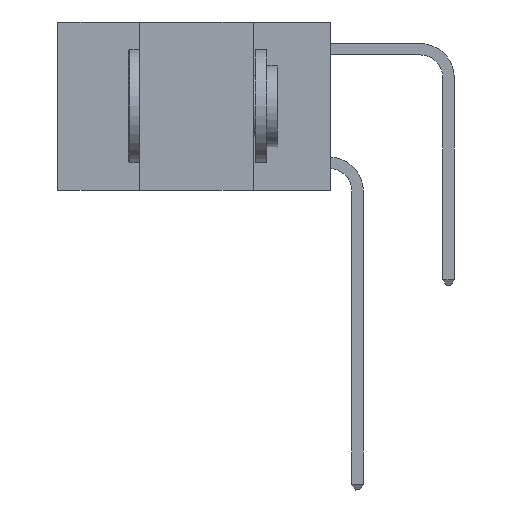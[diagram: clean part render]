
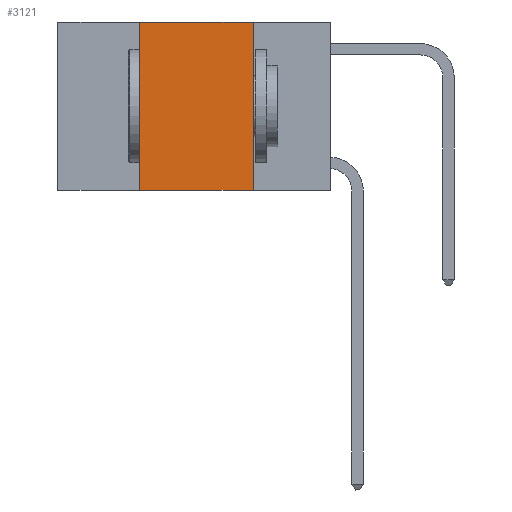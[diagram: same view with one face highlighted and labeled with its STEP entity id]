
A CAD part, left-side view. The second image highlights one B-rep face of the part: STEP entity #3121.
In plain terms, the highlighted planar face has unit normal (-1, 0, 0).
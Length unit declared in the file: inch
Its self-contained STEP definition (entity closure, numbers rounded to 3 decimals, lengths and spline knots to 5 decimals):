
#810 = CARTESIAN_POINT ( 'NONE',  ( 0., 0.6, -0.37 ) ) ;
#1307 = CARTESIAN_POINT ( 'NONE',  ( 0., 0.6, 0. ) ) ;
#1348 = DIRECTION ( 'NONE',  ( 0., 0., -1. ) ) ;
#2406 = EDGE_CURVE ( 'NONE', #4615, #10419, #14867, .T. ) ;
#2535 = PLANE ( 'NONE',  #10834 ) ;
#2639 = DIRECTION ( 'NONE',  ( 0., -1., 0. ) ) ;
#2651 = LINE ( 'NONE', #3707, #6225 ) ;
#2678 = VERTEX_POINT ( 'NONE', #16048 ) ;
#2794 = FACE_OUTER_BOUND ( 'NONE', #12651, .T. ) ;
#3121 = ADVANCED_FACE ( 'NONE', ( #2794 ), #2535, .F. ) ;
#3669 = DIRECTION ( 'NONE',  ( 1., 0., 0. ) ) ;
#3707 = CARTESIAN_POINT ( 'NONE',  ( 0., 0.17, 0. ) ) ;
#4524 = ORIENTED_EDGE ( 'NONE', *, *, #16235, .F. ) ;
#4615 = VERTEX_POINT ( 'NONE', #12975 ) ;
#4662 = ORIENTED_EDGE ( 'NONE', *, *, #15042, .F. ) ;
#5864 = DIRECTION ( 'NONE',  ( 0., 0., -1. ) ) ;
#6085 = CARTESIAN_POINT ( 'NONE',  ( 0., 0.42, 0. ) ) ;
#6225 = VECTOR ( 'NONE', #1348, 39.37008 ) ;
#6996 = LINE ( 'NONE', #810, #7186 ) ;
#7186 = VECTOR ( 'NONE', #13568, 39.37008 ) ;
#8401 = ORIENTED_EDGE ( 'NONE', *, *, #11267, .T. ) ;
#8608 = VERTEX_POINT ( 'NONE', #12066 ) ;
#9026 = CARTESIAN_POINT ( 'NONE',  ( 0., 0.42, 0. ) ) ;
#9897 = LINE ( 'NONE', #1307, #12463 ) ;
#10419 = VERTEX_POINT ( 'NONE', #6085 ) ;
#10834 = AXIS2_PLACEMENT_3D ( 'NONE', #15096, #3669, #5864 ) ;
#11267 = EDGE_CURVE ( 'NONE', #4615, #2678, #6996, .T. ) ;
#11483 = DIRECTION ( 'NONE',  ( 0., 0., 1. ) ) ;
#12066 = CARTESIAN_POINT ( 'NONE',  ( 0., 0.17, 0. ) ) ;
#12463 = VECTOR ( 'NONE', #2639, 39.37008 ) ;
#12651 = EDGE_LOOP ( 'NONE', ( #4662, #4524, #13778, #8401 ) ) ;
#12975 = CARTESIAN_POINT ( 'NONE',  ( 0., 0.42, -0.37 ) ) ;
#13568 = DIRECTION ( 'NONE',  ( 0., -1., 0. ) ) ;
#13778 = ORIENTED_EDGE ( 'NONE', *, *, #2406, .F. ) ;
#14252 = VECTOR ( 'NONE', #11483, 39.37008 ) ;
#14867 = LINE ( 'NONE', #9026, #14252 ) ;
#15042 = EDGE_CURVE ( 'NONE', #8608, #2678, #2651, .T. ) ;
#15096 = CARTESIAN_POINT ( 'NONE',  ( 0., 0.6, 0. ) ) ;
#16048 = CARTESIAN_POINT ( 'NONE',  ( 0., 0.17, -0.37 ) ) ;
#16235 = EDGE_CURVE ( 'NONE', #10419, #8608, #9897, .T. ) ;
